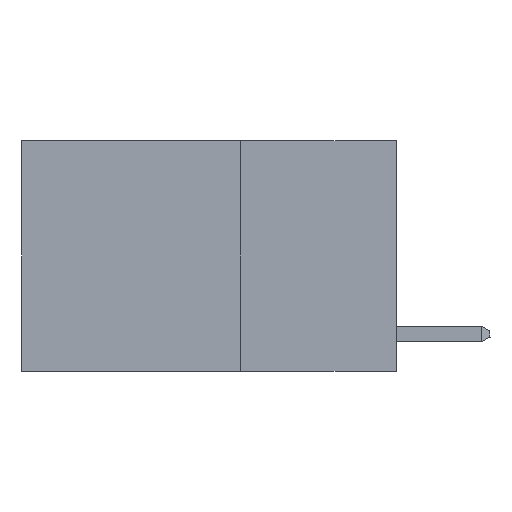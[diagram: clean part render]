
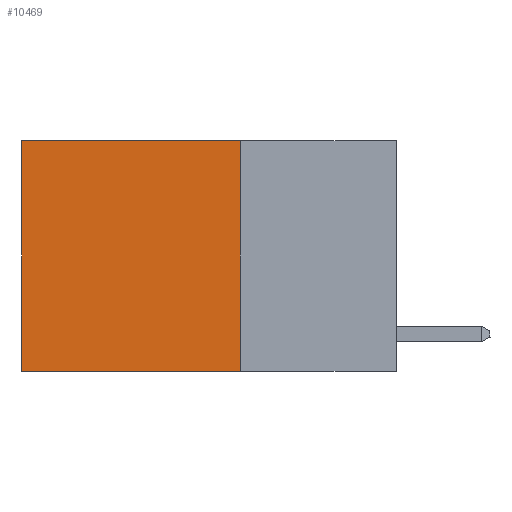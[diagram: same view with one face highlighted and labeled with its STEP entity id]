
A CAD part, left-side view. The second image highlights one B-rep face of the part: STEP entity #10469.
In plain terms, the highlighted planar face has unit normal (-1, 0, 0).
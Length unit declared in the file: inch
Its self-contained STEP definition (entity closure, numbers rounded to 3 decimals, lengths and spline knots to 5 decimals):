
#145 = EDGE_CURVE ( 'NONE', #7111, #8531, #12101, .T. ) ;
#992 = AXIS2_PLACEMENT_3D ( 'NONE', #10125, #11033, #5406 ) ;
#1800 = VECTOR ( 'NONE', #8104, 39.37008 ) ;
#1852 = EDGE_LOOP ( 'NONE', ( #2611, #5725, #2535, #5181 ) ) ;
#1889 = EDGE_CURVE ( 'NONE', #11404, #7331, #7557, .T. ) ;
#1915 = DIRECTION ( 'NONE',  ( 0., 1., 0. ) ) ;
#2535 = ORIENTED_EDGE ( 'NONE', *, *, #1889, .F. ) ;
#2611 = ORIENTED_EDGE ( 'NONE', *, *, #145, .T. ) ;
#2642 = EDGE_CURVE ( 'NONE', #11404, #7111, #9320, .T. ) ;
#3041 = CARTESIAN_POINT ( 'NONE',  ( 0.2625, 0.25, 0. ) ) ;
#3179 = EDGE_CURVE ( 'NONE', #7331, #8531, #9390, .T. ) ;
#3331 = CARTESIAN_POINT ( 'NONE',  ( 0.2625, 0.6, -0.37 ) ) ;
#3496 = PLANE ( 'NONE',  #992 ) ;
#3692 = CARTESIAN_POINT ( 'NONE',  ( 0.2625, 0.25, 0. ) ) ;
#3861 = CARTESIAN_POINT ( 'NONE',  ( 0.2625, 0.25, -0.37 ) ) ;
#4904 = CARTESIAN_POINT ( 'NONE',  ( 0.2625, 0.25, 0. ) ) ;
#5181 = ORIENTED_EDGE ( 'NONE', *, *, #2642, .T. ) ;
#5406 = DIRECTION ( 'NONE',  ( 0., 0., -1. ) ) ;
#5725 = ORIENTED_EDGE ( 'NONE', *, *, #3179, .F. ) ;
#6785 = VECTOR ( 'NONE', #7687, 39.37008 ) ;
#7111 = VERTEX_POINT ( 'NONE', #7355 ) ;
#7331 = VERTEX_POINT ( 'NONE', #3861 ) ;
#7355 = CARTESIAN_POINT ( 'NONE',  ( 0.2625, 0.6, 0. ) ) ;
#7557 = LINE ( 'NONE', #3041, #7860 ) ;
#7687 = DIRECTION ( 'NONE',  ( 0., 1., 0. ) ) ;
#7860 = VECTOR ( 'NONE', #9673, 39.37008 ) ;
#8104 = DIRECTION ( 'NONE',  ( 0., 0., -1. ) ) ;
#8531 = VERTEX_POINT ( 'NONE', #3331 ) ;
#8615 = FACE_OUTER_BOUND ( 'NONE', #1852, .T. ) ;
#9059 = CARTESIAN_POINT ( 'NONE',  ( 0.2625, 0.6, 0. ) ) ;
#9320 = LINE ( 'NONE', #4904, #6785 ) ;
#9390 = LINE ( 'NONE', #10399, #11537 ) ;
#9673 = DIRECTION ( 'NONE',  ( 0., 0., -1. ) ) ;
#10125 = CARTESIAN_POINT ( 'NONE',  ( 0.2625, 0.25, 0. ) ) ;
#10399 = CARTESIAN_POINT ( 'NONE',  ( 0.2625, 0.25, -0.37 ) ) ;
#10469 = ADVANCED_FACE ( 'NONE', ( #8615 ), #3496, .F. ) ;
#11033 = DIRECTION ( 'NONE',  ( 1., 0., 0. ) ) ;
#11404 = VERTEX_POINT ( 'NONE', #3692 ) ;
#11537 = VECTOR ( 'NONE', #1915, 39.37008 ) ;
#12101 = LINE ( 'NONE', #9059, #1800 ) ;
